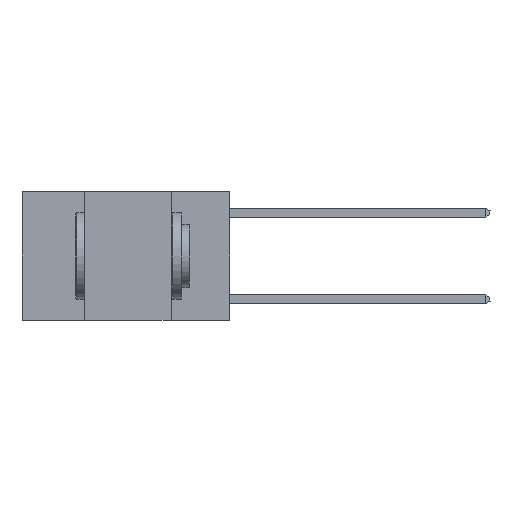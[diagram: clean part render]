
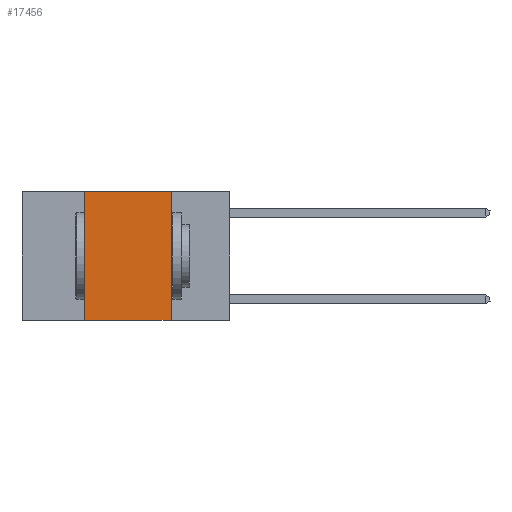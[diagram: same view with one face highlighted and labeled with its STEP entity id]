
A CAD part, left-side view. The second image highlights one B-rep face of the part: STEP entity #17456.
In plain terms, the highlighted planar face has unit normal (-1, 0, 0).
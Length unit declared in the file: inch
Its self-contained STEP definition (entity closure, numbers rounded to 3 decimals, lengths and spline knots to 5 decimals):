
#325 = DIRECTION ( 'NONE',  ( 1., 0., 0. ) ) ;
#637 = CARTESIAN_POINT ( 'NONE',  ( 0., 0.42, -0.37 ) ) ;
#1920 = CARTESIAN_POINT ( 'NONE',  ( 0., 0.17, -0.37 ) ) ;
#2427 = VECTOR ( 'NONE', #7005, 39.37008 ) ;
#5788 = LINE ( 'NONE', #18679, #9537 ) ;
#6078 = CARTESIAN_POINT ( 'NONE',  ( 0., 0.42, 0. ) ) ;
#6096 = EDGE_CURVE ( 'NONE', #7016, #14338, #5788, .T. ) ;
#6189 = LINE ( 'NONE', #6078, #19510 ) ;
#6485 = CARTESIAN_POINT ( 'NONE',  ( 0., 0.6, 0. ) ) ;
#7005 = DIRECTION ( 'NONE',  ( 0., -1., 0. ) ) ;
#7016 = VERTEX_POINT ( 'NONE', #7089 ) ;
#7089 = CARTESIAN_POINT ( 'NONE',  ( 0., 0.17, 0. ) ) ;
#7191 = EDGE_CURVE ( 'NONE', #12188, #14338, #7944, .T. ) ;
#7571 = DIRECTION ( 'NONE',  ( 0., 0., 1. ) ) ;
#7809 = EDGE_LOOP ( 'NONE', ( #11733, #11330, #12669, #19347 ) ) ;
#7944 = LINE ( 'NONE', #9641, #11919 ) ;
#8597 = LINE ( 'NONE', #9009, #2427 ) ;
#9009 = CARTESIAN_POINT ( 'NONE',  ( 0., 0.6, 0. ) ) ;
#9537 = VECTOR ( 'NONE', #15634, 39.37008 ) ;
#9641 = CARTESIAN_POINT ( 'NONE',  ( 0., 0.6, -0.37 ) ) ;
#11330 = ORIENTED_EDGE ( 'NONE', *, *, #12027, .F. ) ;
#11733 = ORIENTED_EDGE ( 'NONE', *, *, #6096, .F. ) ;
#11919 = VECTOR ( 'NONE', #15862, 39.37008 ) ;
#12027 = EDGE_CURVE ( 'NONE', #18539, #7016, #8597, .T. ) ;
#12188 = VERTEX_POINT ( 'NONE', #637 ) ;
#12669 = ORIENTED_EDGE ( 'NONE', *, *, #15409, .F. ) ;
#13357 = DIRECTION ( 'NONE',  ( 0., 0., -1. ) ) ;
#14338 = VERTEX_POINT ( 'NONE', #1920 ) ;
#14746 = PLANE ( 'NONE',  #17581 ) ;
#15409 = EDGE_CURVE ( 'NONE', #12188, #18539, #6189, .T. ) ;
#15634 = DIRECTION ( 'NONE',  ( 0., 0., -1. ) ) ;
#15862 = DIRECTION ( 'NONE',  ( 0., -1., 0. ) ) ;
#17456 = ADVANCED_FACE ( 'NONE', ( #18192 ), #14746, .F. ) ;
#17581 = AXIS2_PLACEMENT_3D ( 'NONE', #6485, #325, #13357 ) ;
#18192 = FACE_OUTER_BOUND ( 'NONE', #7809, .T. ) ;
#18219 = CARTESIAN_POINT ( 'NONE',  ( 0., 0.42, 0. ) ) ;
#18539 = VERTEX_POINT ( 'NONE', #18219 ) ;
#18679 = CARTESIAN_POINT ( 'NONE',  ( 0., 0.17, 0. ) ) ;
#19347 = ORIENTED_EDGE ( 'NONE', *, *, #7191, .T. ) ;
#19510 = VECTOR ( 'NONE', #7571, 39.37008 ) ;
